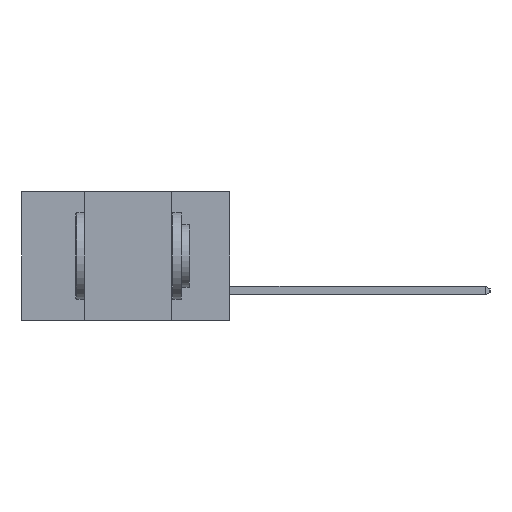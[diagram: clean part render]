
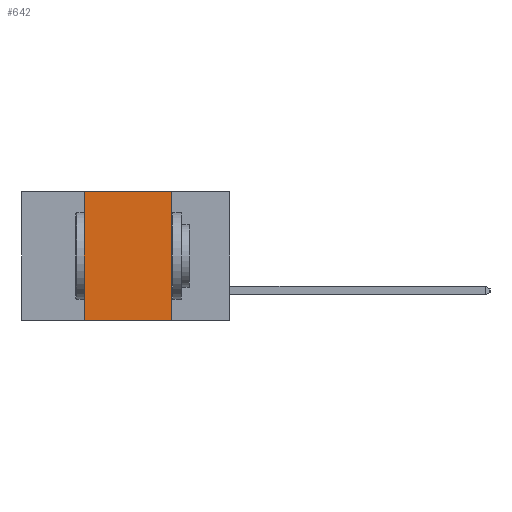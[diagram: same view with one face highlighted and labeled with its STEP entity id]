
A CAD part, left-side view. The second image highlights one B-rep face of the part: STEP entity #642.
In plain terms, the highlighted planar face has unit normal (-1, 0, 0).
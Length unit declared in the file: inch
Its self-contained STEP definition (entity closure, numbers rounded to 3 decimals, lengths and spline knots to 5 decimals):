
#267 = LINE ( 'NONE', #9095, #5391 ) ;
#642 = ADVANCED_FACE ( 'NONE', ( #11643 ), #21198, .F. ) ;
#1537 = LINE ( 'NONE', #14918, #10105 ) ;
#3135 = ORIENTED_EDGE ( 'NONE', *, *, #19665, .F. ) ;
#3353 = EDGE_LOOP ( 'NONE', ( #19640, #3135, #7662, #16764 ) ) ;
#4033 = VECTOR ( 'NONE', #13646, 39.37008 ) ;
#4062 = VECTOR ( 'NONE', #9672, 39.37008 ) ;
#4901 = VERTEX_POINT ( 'NONE', #5695 ) ;
#5391 = VECTOR ( 'NONE', #19234, 39.37008 ) ;
#5695 = CARTESIAN_POINT ( 'NONE',  ( 0., 0.17, -0.37 ) ) ;
#7662 = ORIENTED_EDGE ( 'NONE', *, *, #19893, .F. ) ;
#7941 = CARTESIAN_POINT ( 'NONE',  ( 0., 0.42, -0.37 ) ) ;
#8111 = VERTEX_POINT ( 'NONE', #13422 ) ;
#8537 = LINE ( 'NONE', #13675, #4033 ) ;
#9095 = CARTESIAN_POINT ( 'NONE',  ( 0., 0.6, 0. ) ) ;
#9672 = DIRECTION ( 'NONE',  ( 0., 0., 1. ) ) ;
#10105 = VECTOR ( 'NONE', #14224, 39.37008 ) ;
#10769 = CARTESIAN_POINT ( 'NONE',  ( 0., 0.17, 0. ) ) ;
#11554 = CARTESIAN_POINT ( 'NONE',  ( 0., 0.42, 0. ) ) ;
#11643 = FACE_OUTER_BOUND ( 'NONE', #3353, .T. ) ;
#12721 = EDGE_CURVE ( 'NONE', #8111, #4901, #8537, .T. ) ;
#13422 = CARTESIAN_POINT ( 'NONE',  ( 0., 0.42, -0.37 ) ) ;
#13646 = DIRECTION ( 'NONE',  ( 0., -1., 0. ) ) ;
#13675 = CARTESIAN_POINT ( 'NONE',  ( 0., 0.6, -0.37 ) ) ;
#13972 = EDGE_CURVE ( 'NONE', #17761, #4901, #1537, .T. ) ;
#14224 = DIRECTION ( 'NONE',  ( 0., 0., -1. ) ) ;
#14907 = AXIS2_PLACEMENT_3D ( 'NONE', #21338, #20470, #21342 ) ;
#14918 = CARTESIAN_POINT ( 'NONE',  ( 0., 0.17, -0.37 ) ) ;
#16764 = ORIENTED_EDGE ( 'NONE', *, *, #12721, .T. ) ;
#17679 = LINE ( 'NONE', #7941, #4062 ) ;
#17761 = VERTEX_POINT ( 'NONE', #10769 ) ;
#18087 = VERTEX_POINT ( 'NONE', #11554 ) ;
#19234 = DIRECTION ( 'NONE',  ( 0., -1., 0. ) ) ;
#19640 = ORIENTED_EDGE ( 'NONE', *, *, #13972, .F. ) ;
#19665 = EDGE_CURVE ( 'NONE', #18087, #17761, #267, .T. ) ;
#19893 = EDGE_CURVE ( 'NONE', #8111, #18087, #17679, .T. ) ;
#20470 = DIRECTION ( 'NONE',  ( 1., 0., 0. ) ) ;
#21198 = PLANE ( 'NONE',  #14907 ) ;
#21338 = CARTESIAN_POINT ( 'NONE',  ( 0., 0.6, 0. ) ) ;
#21342 = DIRECTION ( 'NONE',  ( 0., 0., -1. ) ) ;
